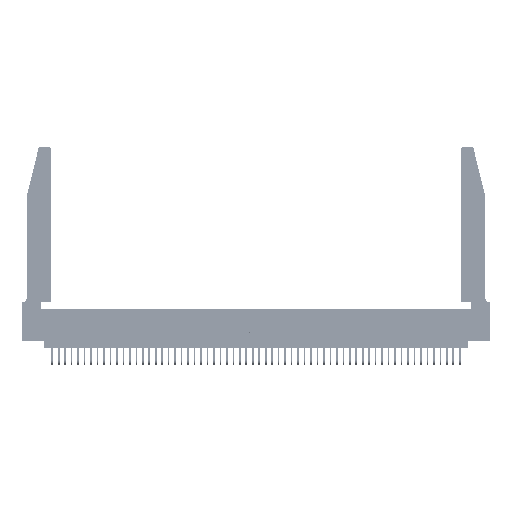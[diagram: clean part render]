
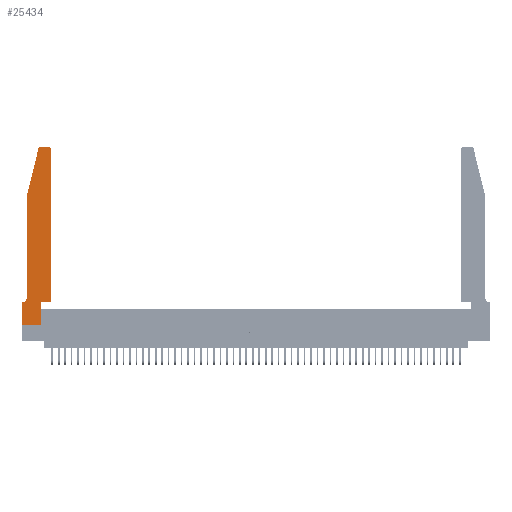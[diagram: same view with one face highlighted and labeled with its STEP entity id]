
A CAD part, top view. The second image highlights one B-rep face of the part: STEP entity #25434.
In plain terms, the highlighted planar face has unit normal (0, 0, 1).
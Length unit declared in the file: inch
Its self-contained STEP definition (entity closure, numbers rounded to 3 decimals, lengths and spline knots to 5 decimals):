
#155 = ORIENTED_EDGE ( 'NONE', *, *, #50670, .T. ) ;
#267 = ORIENTED_EDGE ( 'NONE', *, *, #20268, .T. ) ;
#1018 = DIRECTION ( 'NONE',  ( 0., 0., 1. ) ) ;
#1975 = EDGE_CURVE ( 'NONE', #8039, #38652, #26167, .T. ) ;
#2310 = DIRECTION ( 'NONE',  ( 0., 0., 1. ) ) ;
#2822 = AXIS2_PLACEMENT_3D ( 'NONE', #33975, #8895, #4502 ) ;
#3474 = DIRECTION ( 'NONE',  ( -1., 0., 0. ) ) ;
#4234 = CARTESIAN_POINT ( 'NONE',  ( 0., 0.35, 0.37 ) ) ;
#4502 = DIRECTION ( 'NONE',  ( -1., 0., 0. ) ) ;
#5345 = CARTESIAN_POINT ( 'NONE',  ( 0.4505, 0.35, 0.37 ) ) ;
#5696 = LINE ( 'NONE', #50170, #43469 ) ;
#5851 = LINE ( 'NONE', #9378, #46219 ) ;
#6195 = CARTESIAN_POINT ( 'NONE',  ( 0.284, 2.75, 0.37 ) ) ;
#8039 = VERTEX_POINT ( 'NONE', #6195 ) ;
#8895 = DIRECTION ( 'NONE',  ( 0., 0., -1. ) ) ;
#9155 = CIRCLE ( 'NONE', #33098, 0.03 ) ;
#9378 = CARTESIAN_POINT ( 'NONE',  ( 0.2605, 2.75, 0.37 ) ) ;
#10330 = CARTESIAN_POINT ( 'NONE',  ( 0.2865, 0.35, 0.37 ) ) ;
#10463 = VERTEX_POINT ( 'NONE', #41387 ) ;
#10504 = CARTESIAN_POINT ( 'NONE',  ( 0.0055, 0.35, 0.37 ) ) ;
#10664 = EDGE_CURVE ( 'NONE', #12418, #14675, #52168, .T. ) ;
#11482 = CARTESIAN_POINT ( 'NONE',  ( 0., 0., 0.37 ) ) ;
#12418 = VERTEX_POINT ( 'NONE', #46300 ) ;
#12679 = DIRECTION ( 'NONE',  ( 1., 0., 0. ) ) ;
#13075 = VECTOR ( 'NONE', #22509, 39.37008 ) ;
#14672 = LINE ( 'NONE', #36563, #21823 ) ;
#14675 = VERTEX_POINT ( 'NONE', #11482 ) ;
#15952 = CARTESIAN_POINT ( 'NONE',  ( 0.4505, 0.35, 0.37 ) ) ;
#17589 = CARTESIAN_POINT ( 'NONE',  ( 0.4205, 2.72, 0.37 ) ) ;
#18543 = VERTEX_POINT ( 'NONE', #29361 ) ;
#18685 = EDGE_CURVE ( 'NONE', #21977, #27953, #28541, .T. ) ;
#18992 = CARTESIAN_POINT ( 'NONE',  ( 0., 0., 0.37 ) ) ;
#20144 = DIRECTION ( 'NONE',  ( 1., 0., 0. ) ) ;
#20268 = EDGE_CURVE ( 'NONE', #36888, #12418, #14672, .T. ) ;
#20728 = ORIENTED_EDGE ( 'NONE', *, *, #50983, .T. ) ;
#21161 = DIRECTION ( 'NONE',  ( 0., 0., 1. ) ) ;
#21728 = EDGE_CURVE ( 'NONE', #38652, #46951, #35313, .T. ) ;
#21823 = VECTOR ( 'NONE', #3474, 39.37008 ) ;
#21914 = DIRECTION ( 'NONE',  ( -1., 0., 0. ) ) ;
#21977 = VERTEX_POINT ( 'NONE', #15952 ) ;
#22509 = DIRECTION ( 'NONE',  ( 0., 1., 0. ) ) ;
#22700 = CARTESIAN_POINT ( 'NONE',  ( 0.25487, 2.72718, 0.37 ) ) ;
#23143 = CIRCLE ( 'NONE', #2822, 0.07 ) ;
#24103 = LINE ( 'NONE', #10330, #13075 ) ;
#25434 = ADVANCED_FACE ( 'NONE', ( #26910 ), #33507, .T. ) ;
#25883 = DIRECTION ( 'NONE',  ( 0., -1., 0. ) ) ;
#25994 = LINE ( 'NONE', #18992, #38358 ) ;
#26167 = CIRCLE ( 'NONE', #35608, 0.03 ) ;
#26219 = CARTESIAN_POINT ( 'NONE',  ( 0.0755, 2., 0.37 ) ) ;
#26910 = FACE_OUTER_BOUND ( 'NONE', #34823, .T. ) ;
#27502 = VECTOR ( 'NONE', #46632, 39.37008 ) ;
#27953 = VERTEX_POINT ( 'NONE', #50689 ) ;
#27974 = VERTEX_POINT ( 'NONE', #38113 ) ;
#28466 = AXIS2_PLACEMENT_3D ( 'NONE', #4234, #21161, #33871 ) ;
#28514 = DIRECTION ( 'NONE',  ( 1., 0., 0. ) ) ;
#28541 = LINE ( 'NONE', #5345, #48079 ) ;
#29361 = CARTESIAN_POINT ( 'NONE',  ( 0.0755, 0.42, 0.37 ) ) ;
#31577 = ORIENTED_EDGE ( 'NONE', *, *, #18685, .T. ) ;
#33098 = AXIS2_PLACEMENT_3D ( 'NONE', #17589, #1018, #12679 ) ;
#33507 = PLANE ( 'NONE',  #28466 ) ;
#33871 = DIRECTION ( 'NONE',  ( 1., 0., 0. ) ) ;
#33975 = CARTESIAN_POINT ( 'NONE',  ( 0.0055, 0.42, 0.37 ) ) ;
#34368 = ORIENTED_EDGE ( 'NONE', *, *, #10664, .T. ) ;
#34823 = EDGE_LOOP ( 'NONE', ( #44458, #42741, #37789, #38217, #53103, #267, #34368, #45536, #155, #42498, #31577, #20728 ) ) ;
#35313 = LINE ( 'NONE', #42450, #27502 ) ;
#35388 = CARTESIAN_POINT ( 'NONE',  ( 0.284, 2.72, 0.37 ) ) ;
#35608 = AXIS2_PLACEMENT_3D ( 'NONE', #35388, #2310, #20144 ) ;
#36563 = CARTESIAN_POINT ( 'NONE',  ( 0.0755, 0.35, 0.37 ) ) ;
#36888 = VERTEX_POINT ( 'NONE', #10504 ) ;
#37789 = ORIENTED_EDGE ( 'NONE', *, *, #21728, .T. ) ;
#38113 = CARTESIAN_POINT ( 'NONE',  ( 0.2865, 0., 0.37 ) ) ;
#38217 = ORIENTED_EDGE ( 'NONE', *, *, #52359, .T. ) ;
#38358 = VECTOR ( 'NONE', #48264, 39.37008 ) ;
#38652 = VERTEX_POINT ( 'NONE', #22700 ) ;
#39142 = DIRECTION ( 'NONE',  ( 0., 1., 0. ) ) ;
#39800 = VECTOR ( 'NONE', #25883, 39.37008 ) ;
#41110 = VECTOR ( 'NONE', #28514, 39.37008 ) ;
#41387 = CARTESIAN_POINT ( 'NONE',  ( 0.2865, 0.35, 0.37 ) ) ;
#41460 = EDGE_CURVE ( 'NONE', #18543, #36888, #23143, .T. ) ;
#42116 = CARTESIAN_POINT ( 'NONE',  ( 0., 0., 0.37 ) ) ;
#42433 = LINE ( 'NONE', #53576, #41110 ) ;
#42450 = CARTESIAN_POINT ( 'NONE',  ( 0.0755, 2., 0.37 ) ) ;
#42498 = ORIENTED_EDGE ( 'NONE', *, *, #47870, .T. ) ;
#42741 = ORIENTED_EDGE ( 'NONE', *, *, #1975, .T. ) ;
#43469 = VECTOR ( 'NONE', #49634, 39.37008 ) ;
#44458 = ORIENTED_EDGE ( 'NONE', *, *, #51151, .T. ) ;
#45536 = ORIENTED_EDGE ( 'NONE', *, *, #51403, .T. ) ;
#46219 = VECTOR ( 'NONE', #21914, 39.37008 ) ;
#46300 = CARTESIAN_POINT ( 'NONE',  ( 0., 0.35, 0.37 ) ) ;
#46632 = DIRECTION ( 'NONE',  ( -0.239, -0.971, 0. ) ) ;
#46951 = VERTEX_POINT ( 'NONE', #26219 ) ;
#47870 = EDGE_CURVE ( 'NONE', #10463, #21977, #42433, .T. ) ;
#48079 = VECTOR ( 'NONE', #39142, 39.37008 ) ;
#48264 = DIRECTION ( 'NONE',  ( 1., 0., 0. ) ) ;
#48471 = VERTEX_POINT ( 'NONE', #49004 ) ;
#49004 = CARTESIAN_POINT ( 'NONE',  ( 0.4205, 2.75, 0.37 ) ) ;
#49634 = DIRECTION ( 'NONE',  ( 0., -1., 0. ) ) ;
#50170 = CARTESIAN_POINT ( 'NONE',  ( 0.0755, 2., 0.37 ) ) ;
#50670 = EDGE_CURVE ( 'NONE', #27974, #10463, #24103, .T. ) ;
#50689 = CARTESIAN_POINT ( 'NONE',  ( 0.4505, 2.72, 0.37 ) ) ;
#50983 = EDGE_CURVE ( 'NONE', #27953, #48471, #9155, .T. ) ;
#51151 = EDGE_CURVE ( 'NONE', #48471, #8039, #5851, .T. ) ;
#51403 = EDGE_CURVE ( 'NONE', #14675, #27974, #25994, .T. ) ;
#52168 = LINE ( 'NONE', #42116, #39800 ) ;
#52359 = EDGE_CURVE ( 'NONE', #46951, #18543, #5696, .T. ) ;
#53103 = ORIENTED_EDGE ( 'NONE', *, *, #41460, .T. ) ;
#53576 = CARTESIAN_POINT ( 'NONE',  ( 0.4505, 0.35, 0.37 ) ) ;
